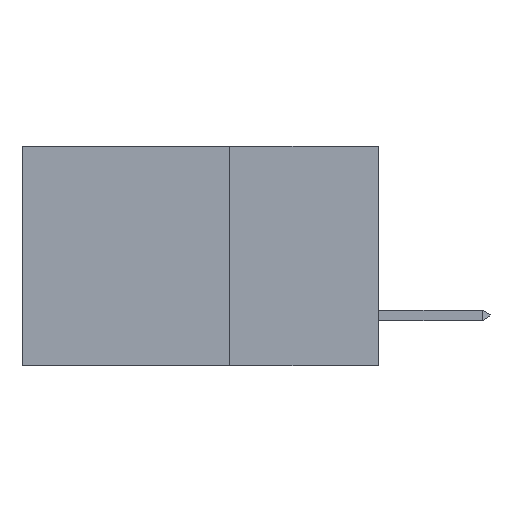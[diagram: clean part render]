
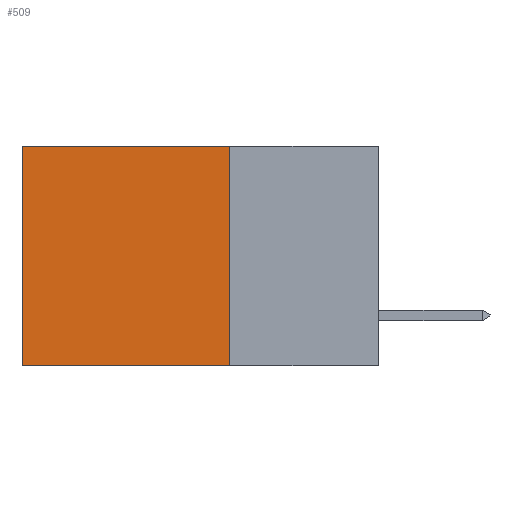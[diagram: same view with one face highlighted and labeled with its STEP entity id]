
A CAD part, left-side view. The second image highlights one B-rep face of the part: STEP entity #509.
In plain terms, the highlighted planar face has unit normal (-1, 0, 0).
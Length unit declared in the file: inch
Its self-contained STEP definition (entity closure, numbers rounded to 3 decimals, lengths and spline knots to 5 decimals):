
#106 = LINE ( 'NONE', #3649, #1495 ) ;
#165 = EDGE_CURVE ( 'NONE', #286, #2990, #8722, .T. ) ;
#217 = AXIS2_PLACEMENT_3D ( 'NONE', #865, #4275, #6135 ) ;
#270 = CARTESIAN_POINT ( 'NONE',  ( 0.2615, 0.6, -0.37 ) ) ;
#286 = VERTEX_POINT ( 'NONE', #2870 ) ;
#386 = VECTOR ( 'NONE', #2554, 39.37008 ) ;
#509 = ADVANCED_FACE ( 'NONE', ( #915 ), #3335, .F. ) ;
#564 = LINE ( 'NONE', #4107, #7889 ) ;
#630 = DIRECTION ( 'NONE',  ( 0., 1., 0. ) ) ;
#865 = CARTESIAN_POINT ( 'NONE',  ( 0.2615, 0.25, -0.37 ) ) ;
#915 = FACE_OUTER_BOUND ( 'NONE', #9019, .T. ) ;
#1495 = VECTOR ( 'NONE', #2577, 39.37008 ) ;
#2117 = ORIENTED_EDGE ( 'NONE', *, *, #2989, .F. ) ;
#2554 = DIRECTION ( 'NONE',  ( 0., 0., -1. ) ) ;
#2577 = DIRECTION ( 'NONE',  ( 0., 0., -1. ) ) ;
#2870 = CARTESIAN_POINT ( 'NONE',  ( 0.2615, 0.6, 0. ) ) ;
#2989 = EDGE_CURVE ( 'NONE', #4328, #3795, #106, .T. ) ;
#2990 = VERTEX_POINT ( 'NONE', #270 ) ;
#3335 = PLANE ( 'NONE',  #217 ) ;
#3649 = CARTESIAN_POINT ( 'NONE',  ( 0.2615, 0.25, -0.37 ) ) ;
#3795 = VERTEX_POINT ( 'NONE', #10350 ) ;
#3814 = EDGE_CURVE ( 'NONE', #3795, #2990, #10295, .T. ) ;
#4020 = ORIENTED_EDGE ( 'NONE', *, *, #165, .T. ) ;
#4107 = CARTESIAN_POINT ( 'NONE',  ( 0.2615, 0.25, 0. ) ) ;
#4275 = DIRECTION ( 'NONE',  ( 1., 0., 0. ) ) ;
#4328 = VERTEX_POINT ( 'NONE', #4543 ) ;
#4543 = CARTESIAN_POINT ( 'NONE',  ( 0.2615, 0.25, 0. ) ) ;
#5595 = EDGE_CURVE ( 'NONE', #4328, #286, #564, .T. ) ;
#6046 = CARTESIAN_POINT ( 'NONE',  ( 0.2615, 0.6, -0.37 ) ) ;
#6085 = DIRECTION ( 'NONE',  ( 0., 1., 0. ) ) ;
#6135 = DIRECTION ( 'NONE',  ( 0., 0., -1. ) ) ;
#6737 = ORIENTED_EDGE ( 'NONE', *, *, #5595, .T. ) ;
#7032 = ORIENTED_EDGE ( 'NONE', *, *, #3814, .F. ) ;
#7889 = VECTOR ( 'NONE', #630, 39.37008 ) ;
#7951 = VECTOR ( 'NONE', #6085, 39.37008 ) ;
#8722 = LINE ( 'NONE', #6046, #386 ) ;
#9019 = EDGE_LOOP ( 'NONE', ( #4020, #7032, #2117, #6737 ) ) ;
#10295 = LINE ( 'NONE', #11070, #7951 ) ;
#10350 = CARTESIAN_POINT ( 'NONE',  ( 0.2615, 0.25, -0.37 ) ) ;
#11070 = CARTESIAN_POINT ( 'NONE',  ( 0.2615, 0.25, -0.37 ) ) ;
